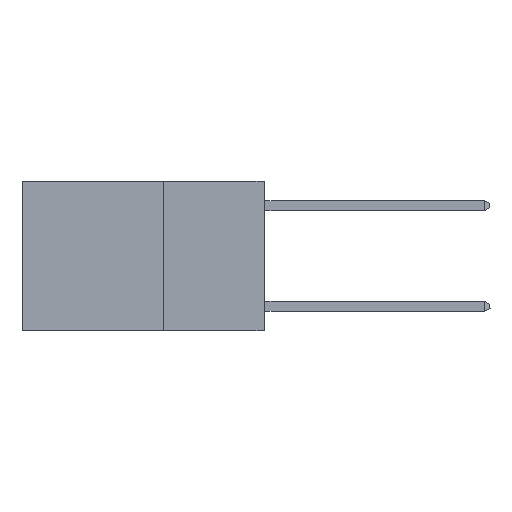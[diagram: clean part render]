
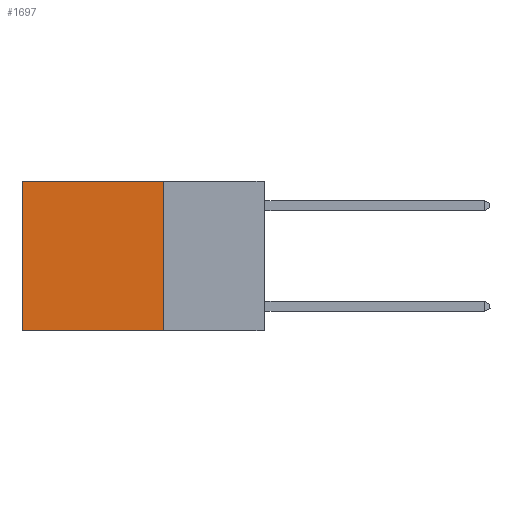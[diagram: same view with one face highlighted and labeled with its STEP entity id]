
A CAD part, left-side view. The second image highlights one B-rep face of the part: STEP entity #1697.
In plain terms, the highlighted planar face has unit normal (-1, 0, 0).
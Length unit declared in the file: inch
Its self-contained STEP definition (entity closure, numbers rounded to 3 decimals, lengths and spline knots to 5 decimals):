
#586 = EDGE_CURVE ( 'NONE', #18929, #10401, #3132, .T. ) ;
#969 = DIRECTION ( 'NONE',  ( 1., 0., 0. ) ) ;
#1697 = ADVANCED_FACE ( 'NONE', ( #7130 ), #10271, .F. ) ;
#1775 = EDGE_CURVE ( 'NONE', #9271, #9976, #8616, .T. ) ;
#3010 = EDGE_CURVE ( 'NONE', #18929, #9271, #14154, .T. ) ;
#3132 = LINE ( 'NONE', #10848, #16249 ) ;
#5724 = DIRECTION ( 'NONE',  ( 0., 0., -1. ) ) ;
#5818 = DIRECTION ( 'NONE',  ( 0., 0., -1. ) ) ;
#5921 = CARTESIAN_POINT ( 'NONE',  ( 0.2625, 0.6, 0. ) ) ;
#6189 = CARTESIAN_POINT ( 'NONE',  ( 0.2625, 0.6, -0.37 ) ) ;
#6412 = CARTESIAN_POINT ( 'NONE',  ( 0.2625, 0.25, -0.37 ) ) ;
#7011 = ORIENTED_EDGE ( 'NONE', *, *, #3010, .T. ) ;
#7130 = FACE_OUTER_BOUND ( 'NONE', #13584, .T. ) ;
#7314 = ORIENTED_EDGE ( 'NONE', *, *, #15576, .F. ) ;
#7686 = ORIENTED_EDGE ( 'NONE', *, *, #586, .F. ) ;
#7813 = DIRECTION ( 'NONE',  ( 0., 1., 0. ) ) ;
#7855 = CARTESIAN_POINT ( 'NONE',  ( 0.2625, 0.25, 0. ) ) ;
#8616 = LINE ( 'NONE', #5921, #18452 ) ;
#8810 = CARTESIAN_POINT ( 'NONE',  ( 0.2625, 0.25, 0. ) ) ;
#9271 = VERTEX_POINT ( 'NONE', #9431 ) ;
#9431 = CARTESIAN_POINT ( 'NONE',  ( 0.2625, 0.6, 0. ) ) ;
#9976 = VERTEX_POINT ( 'NONE', #6189 ) ;
#10271 = PLANE ( 'NONE',  #11819 ) ;
#10401 = VERTEX_POINT ( 'NONE', #11110 ) ;
#10848 = CARTESIAN_POINT ( 'NONE',  ( 0.2625, 0.25, 0. ) ) ;
#11110 = CARTESIAN_POINT ( 'NONE',  ( 0.2625, 0.25, -0.37 ) ) ;
#11819 = AXIS2_PLACEMENT_3D ( 'NONE', #8810, #969, #5724 ) ;
#11948 = DIRECTION ( 'NONE',  ( 0., 0., -1. ) ) ;
#13584 = EDGE_LOOP ( 'NONE', ( #16745, #7314, #7686, #7011 ) ) ;
#13876 = VECTOR ( 'NONE', #17210, 39.37008 ) ;
#14154 = LINE ( 'NONE', #18816, #13876 ) ;
#15576 = EDGE_CURVE ( 'NONE', #10401, #9976, #15590, .T. ) ;
#15590 = LINE ( 'NONE', #6412, #18953 ) ;
#16249 = VECTOR ( 'NONE', #11948, 39.37008 ) ;
#16745 = ORIENTED_EDGE ( 'NONE', *, *, #1775, .T. ) ;
#17210 = DIRECTION ( 'NONE',  ( 0., 1., 0. ) ) ;
#18452 = VECTOR ( 'NONE', #5818, 39.37008 ) ;
#18816 = CARTESIAN_POINT ( 'NONE',  ( 0.2625, 0.25, 0. ) ) ;
#18929 = VERTEX_POINT ( 'NONE', #7855 ) ;
#18953 = VECTOR ( 'NONE', #7813, 39.37008 ) ;
